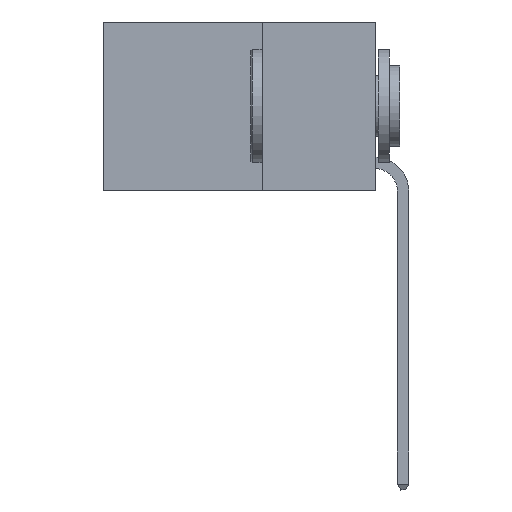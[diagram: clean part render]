
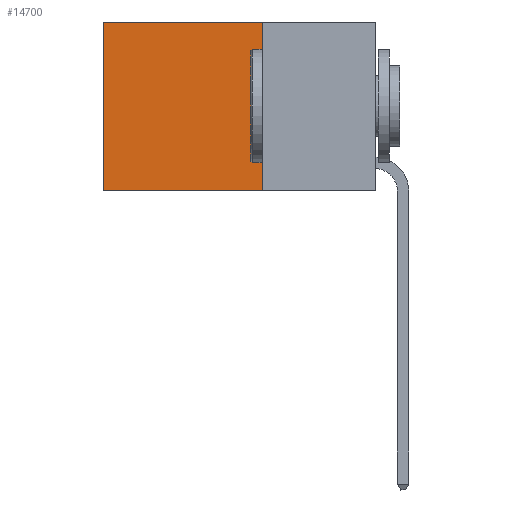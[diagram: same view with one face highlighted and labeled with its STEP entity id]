
A CAD part, left-side view. The second image highlights one B-rep face of the part: STEP entity #14700.
In plain terms, the highlighted planar face has unit normal (-1, 0, 0).
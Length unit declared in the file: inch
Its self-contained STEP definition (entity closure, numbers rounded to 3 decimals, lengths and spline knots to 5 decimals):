
#230 = EDGE_CURVE ( 'NONE', #1788, #7702, #5914, .T. ) ;
#695 = VECTOR ( 'NONE', #9869, 39.37008 ) ;
#1788 = VERTEX_POINT ( 'NONE', #13190 ) ;
#1910 = DIRECTION ( 'NONE',  ( 1., 0., 0. ) ) ;
#1976 = EDGE_LOOP ( 'NONE', ( #16294, #10460, #17015, #4585 ) ) ;
#2084 = CARTESIAN_POINT ( 'NONE',  ( 0.2625, 0.25, 0. ) ) ;
#3008 = CARTESIAN_POINT ( 'NONE',  ( 0.2625, 0.25, -0.37 ) ) ;
#3045 = CARTESIAN_POINT ( 'NONE',  ( 0.2625, 0.6, 0. ) ) ;
#3278 = DIRECTION ( 'NONE',  ( 0., 0., -1. ) ) ;
#3440 = VECTOR ( 'NONE', #7764, 39.37008 ) ;
#4236 = EDGE_CURVE ( 'NONE', #7635, #10423, #6767, .T. ) ;
#4347 = EDGE_CURVE ( 'NONE', #1788, #7635, #12420, .T. ) ;
#4585 = ORIENTED_EDGE ( 'NONE', *, *, #4347, .T. ) ;
#4654 = LINE ( 'NONE', #3008, #14740 ) ;
#5501 = CARTESIAN_POINT ( 'NONE',  ( 0.2625, 0.25, -0.37 ) ) ;
#5914 = LINE ( 'NONE', #15414, #7864 ) ;
#6767 = LINE ( 'NONE', #11901, #3440 ) ;
#7206 = PLANE ( 'NONE',  #17099 ) ;
#7465 = DIRECTION ( 'NONE',  ( 0., 0., -1. ) ) ;
#7635 = VERTEX_POINT ( 'NONE', #3045 ) ;
#7702 = VERTEX_POINT ( 'NONE', #5501 ) ;
#7764 = DIRECTION ( 'NONE',  ( 0., 0., -1. ) ) ;
#7864 = VECTOR ( 'NONE', #3278, 39.37008 ) ;
#8375 = CARTESIAN_POINT ( 'NONE',  ( 0.2625, 0.25, 0. ) ) ;
#9074 = CARTESIAN_POINT ( 'NONE',  ( 0.2625, 0.6, -0.37 ) ) ;
#9869 = DIRECTION ( 'NONE',  ( 0., 1., 0. ) ) ;
#10423 = VERTEX_POINT ( 'NONE', #9074 ) ;
#10460 = ORIENTED_EDGE ( 'NONE', *, *, #11944, .F. ) ;
#11207 = DIRECTION ( 'NONE',  ( 0., 1., 0. ) ) ;
#11901 = CARTESIAN_POINT ( 'NONE',  ( 0.2625, 0.6, 0. ) ) ;
#11944 = EDGE_CURVE ( 'NONE', #7702, #10423, #4654, .T. ) ;
#12420 = LINE ( 'NONE', #8375, #695 ) ;
#13190 = CARTESIAN_POINT ( 'NONE',  ( 0.2625, 0.25, 0. ) ) ;
#14700 = ADVANCED_FACE ( 'NONE', ( #15209 ), #7206, .F. ) ;
#14740 = VECTOR ( 'NONE', #11207, 39.37008 ) ;
#15209 = FACE_OUTER_BOUND ( 'NONE', #1976, .T. ) ;
#15414 = CARTESIAN_POINT ( 'NONE',  ( 0.2625, 0.25, 0. ) ) ;
#16294 = ORIENTED_EDGE ( 'NONE', *, *, #4236, .T. ) ;
#17015 = ORIENTED_EDGE ( 'NONE', *, *, #230, .F. ) ;
#17099 = AXIS2_PLACEMENT_3D ( 'NONE', #2084, #1910, #7465 ) ;
